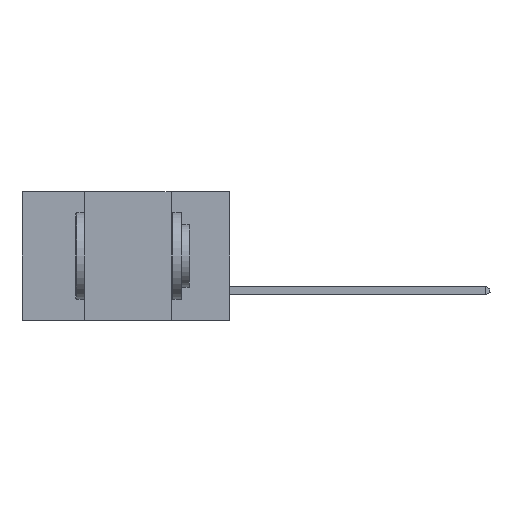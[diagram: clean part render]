
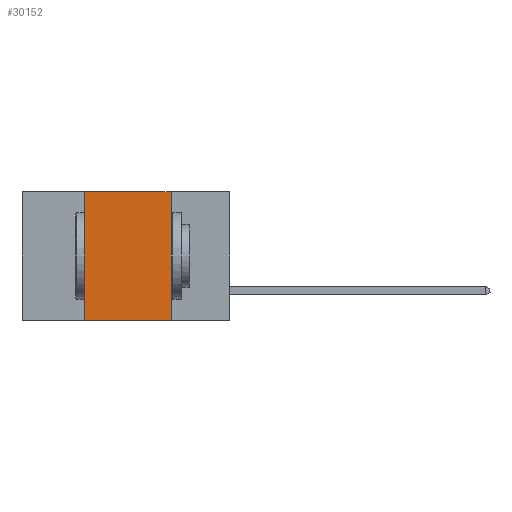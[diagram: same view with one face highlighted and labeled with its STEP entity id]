
A CAD part, left-side view. The second image highlights one B-rep face of the part: STEP entity #30152.
In plain terms, the highlighted planar face has unit normal (-1, 0, 0).
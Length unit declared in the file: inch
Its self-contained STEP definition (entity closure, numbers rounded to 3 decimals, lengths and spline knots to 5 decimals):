
#982 = VECTOR ( 'NONE', #22511, 39.37008 ) ;
#3027 = LINE ( 'NONE', #23294, #24696 ) ;
#3066 = ORIENTED_EDGE ( 'NONE', *, *, #25126, .F. ) ;
#3334 = CARTESIAN_POINT ( 'NONE',  ( 0., 0.42, 0. ) ) ;
#3795 = VERTEX_POINT ( 'NONE', #21626 ) ;
#3841 = VECTOR ( 'NONE', #15433, 39.37008 ) ;
#5138 = VECTOR ( 'NONE', #6082, 39.37008 ) ;
#5539 = FACE_OUTER_BOUND ( 'NONE', #25332, .T. ) ;
#6082 = DIRECTION ( 'NONE',  ( 0., -1., 0. ) ) ;
#6714 = DIRECTION ( 'NONE',  ( 1., 0., 0. ) ) ;
#7021 = DIRECTION ( 'NONE',  ( 0., 0., -1. ) ) ;
#7616 = ORIENTED_EDGE ( 'NONE', *, *, #12313, .F. ) ;
#8975 = LINE ( 'NONE', #30455, #5138 ) ;
#11585 = EDGE_CURVE ( 'NONE', #23134, #20786, #28463, .T. ) ;
#12313 = EDGE_CURVE ( 'NONE', #17382, #3795, #3027, .T. ) ;
#13148 = CARTESIAN_POINT ( 'NONE',  ( 0., 0.6, 0. ) ) ;
#14186 = ORIENTED_EDGE ( 'NONE', *, *, #11585, .F. ) ;
#14590 = AXIS2_PLACEMENT_3D ( 'NONE', #26237, #6714, #7021 ) ;
#14973 = CARTESIAN_POINT ( 'NONE',  ( 0., 0.42, 0. ) ) ;
#15395 = ORIENTED_EDGE ( 'NONE', *, *, #16705, .T. ) ;
#15433 = DIRECTION ( 'NONE',  ( 0., 0., 1. ) ) ;
#16705 = EDGE_CURVE ( 'NONE', #23134, #3795, #8975, .T. ) ;
#17382 = VERTEX_POINT ( 'NONE', #30187 ) ;
#18837 = LINE ( 'NONE', #13148, #982 ) ;
#20786 = VERTEX_POINT ( 'NONE', #14973 ) ;
#21626 = CARTESIAN_POINT ( 'NONE',  ( 0., 0.17, -0.37 ) ) ;
#22121 = CARTESIAN_POINT ( 'NONE',  ( 0., 0.42, -0.37 ) ) ;
#22511 = DIRECTION ( 'NONE',  ( 0., -1., 0. ) ) ;
#23134 = VERTEX_POINT ( 'NONE', #22121 ) ;
#23294 = CARTESIAN_POINT ( 'NONE',  ( 0., 0.17, 0. ) ) ;
#24696 = VECTOR ( 'NONE', #25728, 39.37008 ) ;
#25126 = EDGE_CURVE ( 'NONE', #20786, #17382, #18837, .T. ) ;
#25332 = EDGE_LOOP ( 'NONE', ( #7616, #3066, #14186, #15395 ) ) ;
#25728 = DIRECTION ( 'NONE',  ( 0., 0., -1. ) ) ;
#26237 = CARTESIAN_POINT ( 'NONE',  ( 0., 0.6, 0. ) ) ;
#28463 = LINE ( 'NONE', #3334, #3841 ) ;
#28841 = PLANE ( 'NONE',  #14590 ) ;
#30152 = ADVANCED_FACE ( 'NONE', ( #5539 ), #28841, .F. ) ;
#30187 = CARTESIAN_POINT ( 'NONE',  ( 0., 0.17, 0. ) ) ;
#30455 = CARTESIAN_POINT ( 'NONE',  ( 0., 0.6, -0.37 ) ) ;
